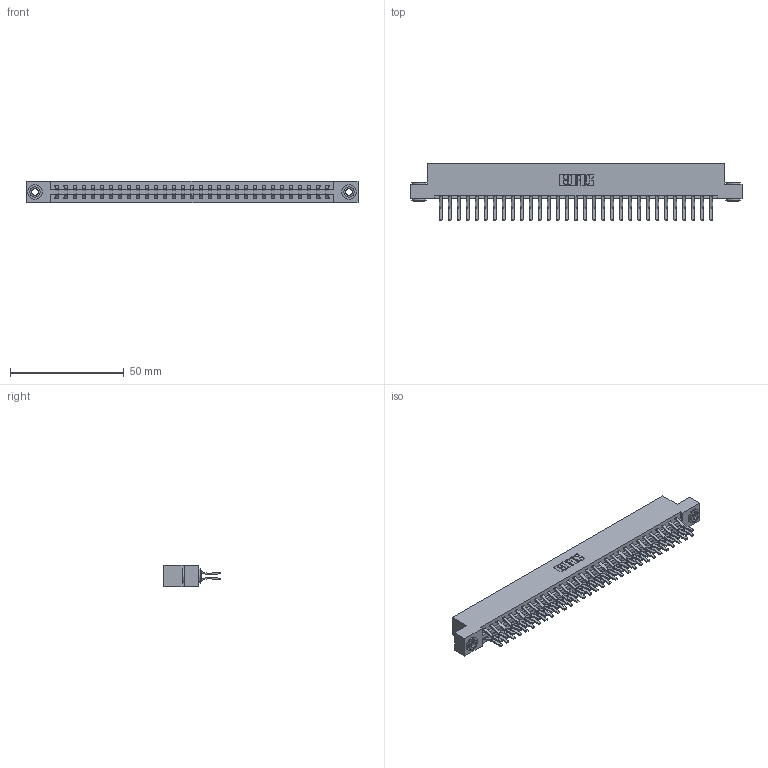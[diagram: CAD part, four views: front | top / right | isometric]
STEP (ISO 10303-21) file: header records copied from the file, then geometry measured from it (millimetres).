
FILE_DESCRIPTION (( 'STEP AP203' ), '1' );
FILE_NAME ('387-062-560-203.STEP', '2018-09-21T06:29:59', ( '' ), ( '' ), 'SwSTEP 2.0', 'SolidWorks 2016', '' );
FILE_SCHEMA (( 'CONFIG_CONTROL_DESIGN' ));
Length unit declared in the file: inch
Products named in the file (4): 387-062-560-203; 337 Part_Flush Mounting Lugs - 0.156 Dia-TH; 345-292-001_560 Tail; 345-250-002_345-250-002-102
Assembly tree (65 placements, depth 2):
  387-062-560-203
    337 Part_Flush Mounting Lugs - 0.156 Dia-TH
    345-292-001_560 Tail  x62
    345-250-002_345-250-002-102  x2
Bounding box: 145.85 x 24.78 x 9.4 mm (x, y, z)
Volume: 15649.9 mm3; surface area: 18985.9 mm2
Topology: 65 solids, 65 shells, 3624 faces, 10741 edges, 7074 vertices
Faces by surface type: plane 2436, cylinder 1180, cone 8
Entity records: 26196 total; most frequent: CARTESIAN_POINT 4397, ORIENTED_EDGE 4326, DIRECTION 3797, EDGE_CURVE 2163, VECTOR 2007, LINE 2007, VERTEX_POINT 1438, AXIS2_PLACEMENT_3D 895
